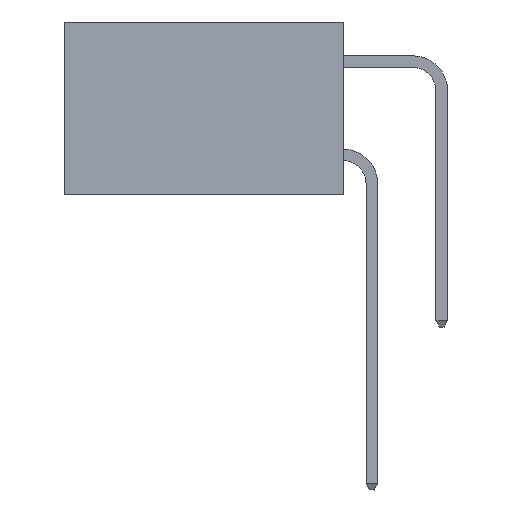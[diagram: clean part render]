
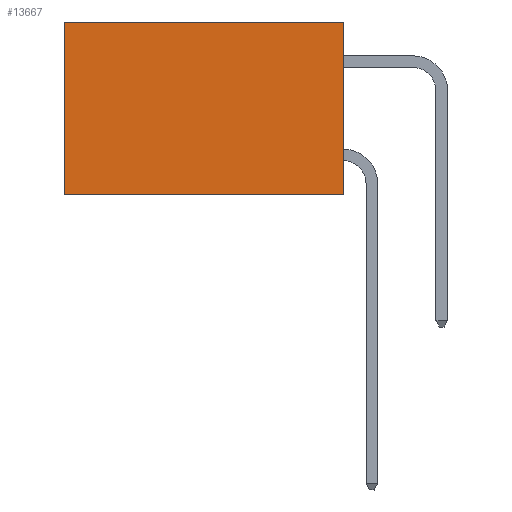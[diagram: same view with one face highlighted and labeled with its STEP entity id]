
A CAD part, left-side view. The second image highlights one B-rep face of the part: STEP entity #13667.
In plain terms, the highlighted planar face has unit normal (-1, 0, 0).
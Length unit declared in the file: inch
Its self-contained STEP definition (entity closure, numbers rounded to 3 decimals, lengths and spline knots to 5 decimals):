
#3935 = PLANE ( 'NONE',  #15909 ) ;
#4058 = VECTOR ( 'NONE', #20098, 39.37008 ) ;
#5314 = CARTESIAN_POINT ( 'NONE',  ( 0.2615, 0., -0.37 ) ) ;
#5779 = CARTESIAN_POINT ( 'NONE',  ( 0.2615, 0., -0.37 ) ) ;
#5820 = DIRECTION ( 'NONE',  ( 1., 0., 0. ) ) ;
#5993 = EDGE_CURVE ( 'NONE', #17784, #19355, #25141, .T. ) ;
#6353 = CARTESIAN_POINT ( 'NONE',  ( 0.2615, 0.6, 0. ) ) ;
#6739 = DIRECTION ( 'NONE',  ( 0., 0., -1. ) ) ;
#9124 = VERTEX_POINT ( 'NONE', #6353 ) ;
#9914 = EDGE_LOOP ( 'NONE', ( #11132, #18778, #16819, #22911 ) ) ;
#10826 = EDGE_CURVE ( 'NONE', #28463, #9124, #25335, .T. ) ;
#11132 = ORIENTED_EDGE ( 'NONE', *, *, #19177, .T. ) ;
#12354 = CARTESIAN_POINT ( 'NONE',  ( 0.2615, 0., 0. ) ) ;
#13667 = ADVANCED_FACE ( 'NONE', ( #17242 ), #3935, .F. ) ;
#14048 = CARTESIAN_POINT ( 'NONE',  ( 0.2615, 0.6, -0.37 ) ) ;
#14221 = EDGE_CURVE ( 'NONE', #28463, #17784, #22609, .T. ) ;
#14651 = DIRECTION ( 'NONE',  ( 0., 0., -1. ) ) ;
#15909 = AXIS2_PLACEMENT_3D ( 'NONE', #16803, #5820, #14651 ) ;
#16041 = CARTESIAN_POINT ( 'NONE',  ( 0.2615, 0., 0. ) ) ;
#16803 = CARTESIAN_POINT ( 'NONE',  ( 0.2615, 0., -0.37 ) ) ;
#16819 = ORIENTED_EDGE ( 'NONE', *, *, #14221, .F. ) ;
#17242 = FACE_OUTER_BOUND ( 'NONE', #9914, .T. ) ;
#17784 = VERTEX_POINT ( 'NONE', #5314 ) ;
#18778 = ORIENTED_EDGE ( 'NONE', *, *, #5993, .F. ) ;
#19177 = EDGE_CURVE ( 'NONE', #9124, #19355, #22819, .T. ) ;
#19355 = VERTEX_POINT ( 'NONE', #25431 ) ;
#20033 = CARTESIAN_POINT ( 'NONE',  ( 0.2615, 0., -0.37 ) ) ;
#20098 = DIRECTION ( 'NONE',  ( 0., 0., -1. ) ) ;
#20573 = DIRECTION ( 'NONE',  ( 0., 1., 0. ) ) ;
#22609 = LINE ( 'NONE', #20033, #23790 ) ;
#22819 = LINE ( 'NONE', #14048, #4058 ) ;
#22911 = ORIENTED_EDGE ( 'NONE', *, *, #10826, .T. ) ;
#23790 = VECTOR ( 'NONE', #6739, 39.37008 ) ;
#25141 = LINE ( 'NONE', #5779, #25869 ) ;
#25335 = LINE ( 'NONE', #12354, #28296 ) ;
#25431 = CARTESIAN_POINT ( 'NONE',  ( 0.2615, 0.6, -0.37 ) ) ;
#25869 = VECTOR ( 'NONE', #27614, 39.37008 ) ;
#27614 = DIRECTION ( 'NONE',  ( 0., 1., 0. ) ) ;
#28296 = VECTOR ( 'NONE', #20573, 39.37008 ) ;
#28463 = VERTEX_POINT ( 'NONE', #16041 ) ;
